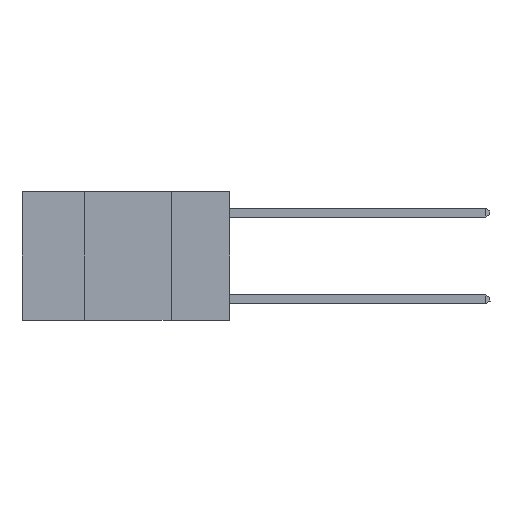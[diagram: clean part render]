
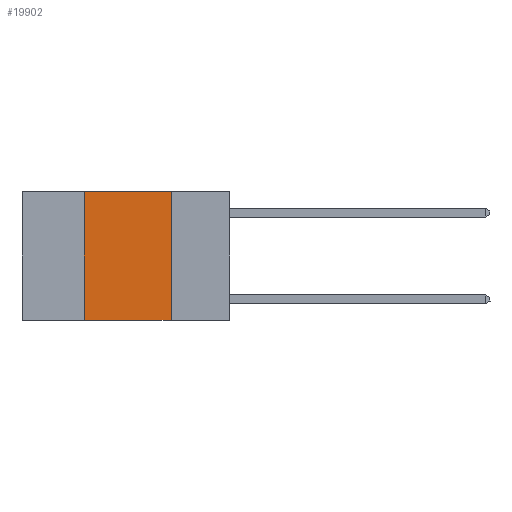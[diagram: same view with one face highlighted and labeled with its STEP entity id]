
A CAD part, left-side view. The second image highlights one B-rep face of the part: STEP entity #19902.
In plain terms, the highlighted planar face has unit normal (-1, 0, 0).
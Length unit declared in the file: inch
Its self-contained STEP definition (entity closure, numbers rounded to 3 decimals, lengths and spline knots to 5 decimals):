
#896 = AXIS2_PLACEMENT_3D ( 'NONE', #7205, #16862, #5393 ) ;
#3476 = PLANE ( 'NONE',  #896 ) ;
#3492 = VERTEX_POINT ( 'NONE', #4986 ) ;
#3524 = CARTESIAN_POINT ( 'NONE',  ( 0., 0.6, 0. ) ) ;
#4986 = CARTESIAN_POINT ( 'NONE',  ( 0., 0.42, 0. ) ) ;
#5393 = DIRECTION ( 'NONE',  ( 0., 0., -1. ) ) ;
#5732 = LINE ( 'NONE', #3524, #10174 ) ;
#6291 = EDGE_CURVE ( 'NONE', #17612, #3492, #17862, .T. ) ;
#7205 = CARTESIAN_POINT ( 'NONE',  ( 0., 0.6, 0. ) ) ;
#9164 = CARTESIAN_POINT ( 'NONE',  ( 0., 0.42, 0. ) ) ;
#9355 = VERTEX_POINT ( 'NONE', #19003 ) ;
#10174 = VECTOR ( 'NONE', #16910, 39.37008 ) ;
#10337 = EDGE_CURVE ( 'NONE', #3492, #9355, #5732, .T. ) ;
#10548 = CARTESIAN_POINT ( 'NONE',  ( 0., 0.17, -0.37 ) ) ;
#10793 = VERTEX_POINT ( 'NONE', #10548 ) ;
#11078 = ORIENTED_EDGE ( 'NONE', *, *, #21912, .T. ) ;
#11205 = ORIENTED_EDGE ( 'NONE', *, *, #11798, .F. ) ;
#11798 = EDGE_CURVE ( 'NONE', #9355, #10793, #19951, .T. ) ;
#13382 = LINE ( 'NONE', #16869, #22231 ) ;
#14345 = VECTOR ( 'NONE', #22658, 39.37008 ) ;
#16862 = DIRECTION ( 'NONE',  ( 1., 0., 0. ) ) ;
#16869 = CARTESIAN_POINT ( 'NONE',  ( 0., 0.6, -0.37 ) ) ;
#16910 = DIRECTION ( 'NONE',  ( 0., -1., 0. ) ) ;
#17083 = FACE_OUTER_BOUND ( 'NONE', #21294, .T. ) ;
#17106 = CARTESIAN_POINT ( 'NONE',  ( 0., 0.17, 0. ) ) ;
#17286 = ORIENTED_EDGE ( 'NONE', *, *, #10337, .F. ) ;
#17472 = ORIENTED_EDGE ( 'NONE', *, *, #6291, .F. ) ;
#17612 = VERTEX_POINT ( 'NONE', #21254 ) ;
#17862 = LINE ( 'NONE', #9164, #22242 ) ;
#18715 = DIRECTION ( 'NONE',  ( 0., 0., 1. ) ) ;
#19003 = CARTESIAN_POINT ( 'NONE',  ( 0., 0.17, 0. ) ) ;
#19902 = ADVANCED_FACE ( 'NONE', ( #17083 ), #3476, .F. ) ;
#19951 = LINE ( 'NONE', #17106, #14345 ) ;
#21254 = CARTESIAN_POINT ( 'NONE',  ( 0., 0.42, -0.37 ) ) ;
#21294 = EDGE_LOOP ( 'NONE', ( #11205, #17286, #17472, #11078 ) ) ;
#21912 = EDGE_CURVE ( 'NONE', #17612, #10793, #13382, .T. ) ;
#22231 = VECTOR ( 'NONE', #22433, 39.37008 ) ;
#22242 = VECTOR ( 'NONE', #18715, 39.37008 ) ;
#22433 = DIRECTION ( 'NONE',  ( 0., -1., 0. ) ) ;
#22658 = DIRECTION ( 'NONE',  ( 0., 0., -1. ) ) ;
